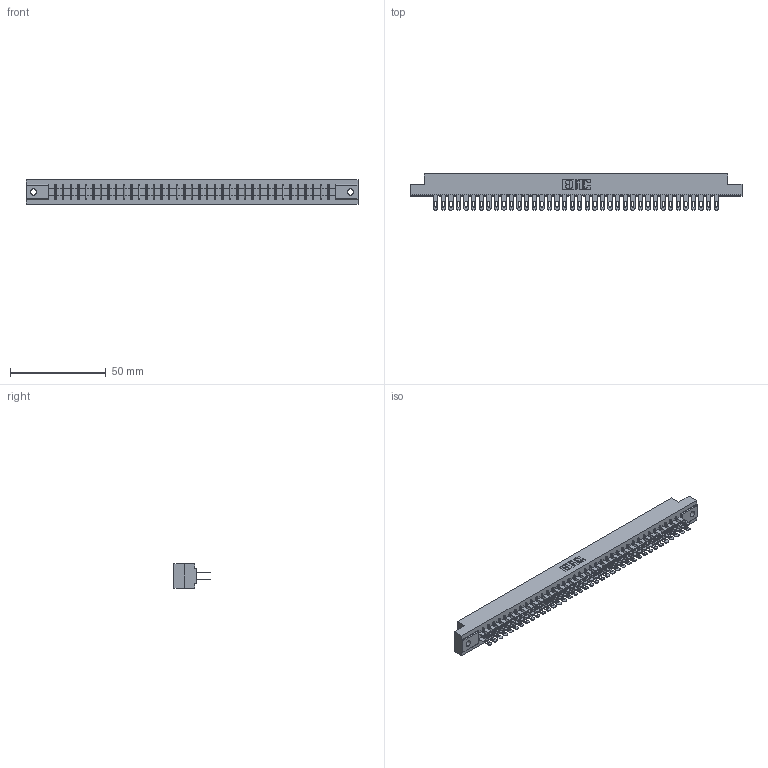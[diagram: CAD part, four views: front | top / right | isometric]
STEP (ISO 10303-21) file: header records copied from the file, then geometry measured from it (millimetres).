
FILE_DESCRIPTION (( 'STEP AP203' ), '1' );
FILE_NAME ('355-076-500-502.STEP', '2019-09-13T13:05:15', ( '' ), ( '' ), 'SwSTEP 2.0', 'SolidWorks 2016', '' );
FILE_SCHEMA (( 'CONFIG_CONTROL_DESIGN' ));
Length unit declared in the file: inch
Products named in the file (3): 305 Part_.128 Dia; 355-076-500-502; 305-290-001_500
Assembly tree (77 placements, depth 2):
  355-076-500-502
    305 Part_.128 Dia
    305-290-001_500  x76
Bounding box: 173.58 x 18.85 x 12.7 mm (x, y, z)
Volume: 17757.6 mm3; surface area: 24558.3 mm2
Topology: 77 solids, 77 shells, 3916 faces, 11222 edges, 7276 vertices
Faces by surface type: plane 2196, cylinder 1568, sphere 152
Entity records: 41655 total; most frequent: CARTESIAN_POINT 6892, ORIENTED_EDGE 6840, DIRECTION 6672, EDGE_CURVE 3420, VECTOR 2760, LINE 2760, VERTEX_POINT 2176, AXIS2_PLACEMENT_3D 1956
